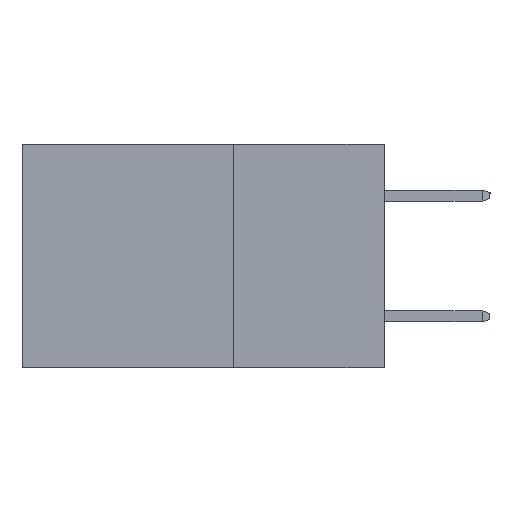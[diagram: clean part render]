
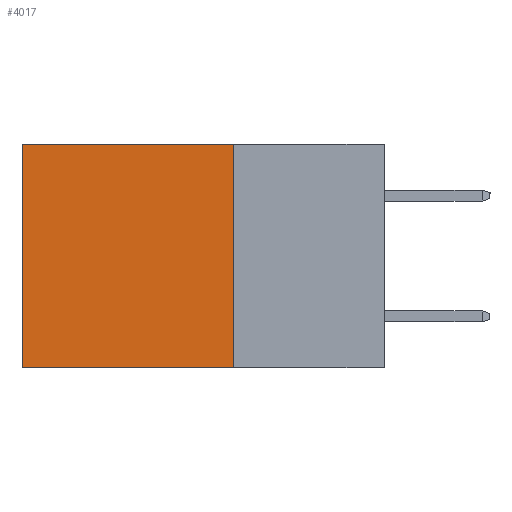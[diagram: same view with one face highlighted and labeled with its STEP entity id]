
A CAD part, left-side view. The second image highlights one B-rep face of the part: STEP entity #4017.
In plain terms, the highlighted planar face has unit normal (-1, 0, 0).
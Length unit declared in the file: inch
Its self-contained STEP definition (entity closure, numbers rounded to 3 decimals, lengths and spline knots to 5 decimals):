
#950 = CARTESIAN_POINT ( 'NONE',  ( 0.2615, 0.6, -0.37 ) ) ;
#1077 = VECTOR ( 'NONE', #14331, 39.37008 ) ;
#1798 = EDGE_CURVE ( 'NONE', #13657, #4145, #14190, .T. ) ;
#1867 = CARTESIAN_POINT ( 'NONE',  ( 0.2615, 0.25, 0. ) ) ;
#2024 = DIRECTION ( 'NONE',  ( 1., 0., 0. ) ) ;
#2438 = ORIENTED_EDGE ( 'NONE', *, *, #15052, .T. ) ;
#2485 = VECTOR ( 'NONE', #12866, 39.37008 ) ;
#2991 = ORIENTED_EDGE ( 'NONE', *, *, #1798, .F. ) ;
#3239 = CARTESIAN_POINT ( 'NONE',  ( 0.2615, 0.25, -0.37 ) ) ;
#4017 = ADVANCED_FACE ( 'NONE', ( #6798 ), #11794, .F. ) ;
#4121 = EDGE_CURVE ( 'NONE', #5690, #13657, #7926, .T. ) ;
#4145 = VERTEX_POINT ( 'NONE', #14231 ) ;
#4178 = CARTESIAN_POINT ( 'NONE',  ( 0.2615, 0.25, 0. ) ) ;
#4301 = CARTESIAN_POINT ( 'NONE',  ( 0.2615, 0.25, -0.37 ) ) ;
#4637 = CARTESIAN_POINT ( 'NONE',  ( 0.2615, 0.25, -0.37 ) ) ;
#5038 = ORIENTED_EDGE ( 'NONE', *, *, #4121, .F. ) ;
#5690 = VERTEX_POINT ( 'NONE', #1867 ) ;
#6798 = FACE_OUTER_BOUND ( 'NONE', #9417, .T. ) ;
#7488 = EDGE_CURVE ( 'NONE', #10039, #4145, #15748, .T. ) ;
#7926 = LINE ( 'NONE', #3239, #2485 ) ;
#8246 = DIRECTION ( 'NONE',  ( 0., 0., -1. ) ) ;
#9417 = EDGE_LOOP ( 'NONE', ( #12234, #2991, #5038, #2438 ) ) ;
#9563 = LINE ( 'NONE', #4178, #1077 ) ;
#10039 = VERTEX_POINT ( 'NONE', #11453 ) ;
#10817 = DIRECTION ( 'NONE',  ( 0., 0., -1. ) ) ;
#11453 = CARTESIAN_POINT ( 'NONE',  ( 0.2615, 0.6, 0. ) ) ;
#11794 = PLANE ( 'NONE',  #15836 ) ;
#12048 = VECTOR ( 'NONE', #10817, 39.37008 ) ;
#12234 = ORIENTED_EDGE ( 'NONE', *, *, #7488, .T. ) ;
#12866 = DIRECTION ( 'NONE',  ( 0., 0., -1. ) ) ;
#13657 = VERTEX_POINT ( 'NONE', #4637 ) ;
#14190 = LINE ( 'NONE', #15399, #15811 ) ;
#14231 = CARTESIAN_POINT ( 'NONE',  ( 0.2615, 0.6, -0.37 ) ) ;
#14331 = DIRECTION ( 'NONE',  ( 0., 1., 0. ) ) ;
#15052 = EDGE_CURVE ( 'NONE', #5690, #10039, #9563, .T. ) ;
#15399 = CARTESIAN_POINT ( 'NONE',  ( 0.2615, 0.25, -0.37 ) ) ;
#15718 = DIRECTION ( 'NONE',  ( 0., 1., 0. ) ) ;
#15748 = LINE ( 'NONE', #950, #12048 ) ;
#15811 = VECTOR ( 'NONE', #15718, 39.37008 ) ;
#15836 = AXIS2_PLACEMENT_3D ( 'NONE', #4301, #2024, #8246 ) ;
